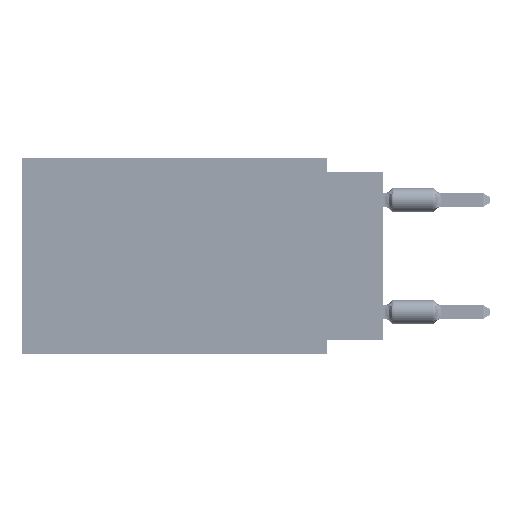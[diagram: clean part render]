
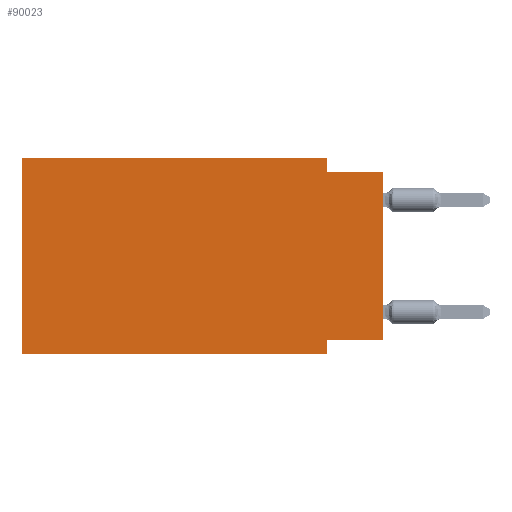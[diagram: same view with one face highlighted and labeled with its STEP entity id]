
A CAD part, left-side view. The second image highlights one B-rep face of the part: STEP entity #90023.
In plain terms, the highlighted planar face has unit normal (-1, 0, 0).
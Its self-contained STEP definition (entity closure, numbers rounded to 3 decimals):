
#874 = DIRECTION ( 'NONE',  ( 0., -1., 0. ) ) ;
#1228 = DIRECTION ( 'NONE',  ( 0., 0., 1. ) ) ;
#2649 = ORIENTED_EDGE ( 'NONE', *, *, #95040, .F. ) ;
#3822 = EDGE_CURVE ( 'NONE', #44511, #113213, #54202, .T. ) ;
#7982 = DIRECTION ( 'NONE',  ( 0., 0., -1. ) ) ;
#8481 = DIRECTION ( 'NONE',  ( 0., 0., -1. ) ) ;
#10222 = CARTESIAN_POINT ( 'NONE',  ( 0., 16.383, 0. ) ) ;
#14307 = LINE ( 'NONE', #70844, #91828 ) ;
#15457 = EDGE_CURVE ( 'NONE', #113213, #62733, #33739, .T. ) ;
#15697 = CARTESIAN_POINT ( 'NONE',  ( 0., 0., -0.635 ) ) ;
#17548 = VERTEX_POINT ( 'NONE', #62936 ) ;
#18003 = VERTEX_POINT ( 'NONE', #44712 ) ;
#18806 = PLANE ( 'NONE',  #70451 ) ;
#21100 = DIRECTION ( 'NONE',  ( 0., -1., 0. ) ) ;
#22506 = ORIENTED_EDGE ( 'NONE', *, *, #78497, .T. ) ;
#24770 = CARTESIAN_POINT ( 'NONE',  ( 0., 2.54, -8.89 ) ) ;
#27828 = FACE_OUTER_BOUND ( 'NONE', #87710, .T. ) ;
#31511 = ORIENTED_EDGE ( 'NONE', *, *, #15457, .F. ) ;
#33739 = LINE ( 'NONE', #15697, #103133 ) ;
#33762 = VERTEX_POINT ( 'NONE', #91388 ) ;
#34558 = VECTOR ( 'NONE', #21100, 1000. ) ;
#36956 = CARTESIAN_POINT ( 'NONE',  ( 0., 16.383, -8.89 ) ) ;
#39013 = VECTOR ( 'NONE', #68711, 1000. ) ;
#40032 = CARTESIAN_POINT ( 'NONE',  ( 0., 2.54, -0.635 ) ) ;
#44511 = VERTEX_POINT ( 'NONE', #113572 ) ;
#44712 = CARTESIAN_POINT ( 'NONE',  ( 0., 2.54, -8.255 ) ) ;
#47925 = ORIENTED_EDGE ( 'NONE', *, *, #105461, .F. ) ;
#52383 = DIRECTION ( 'NONE',  ( 0., -1., 0. ) ) ;
#54202 = LINE ( 'NONE', #90938, #81335 ) ;
#56422 = VERTEX_POINT ( 'NONE', #104288 ) ;
#56747 = LINE ( 'NONE', #103671, #94701 ) ;
#62733 = VERTEX_POINT ( 'NONE', #88961 ) ;
#62936 = CARTESIAN_POINT ( 'NONE',  ( 0., 16.383, 0. ) ) ;
#67404 = VECTOR ( 'NONE', #874, 1000. ) ;
#68711 = DIRECTION ( 'NONE',  ( 0., 0., -1. ) ) ;
#70451 = AXIS2_PLACEMENT_3D ( 'NONE', #91040, #72961, #7982 ) ;
#70844 = CARTESIAN_POINT ( 'NONE',  ( 0., 0., 0. ) ) ;
#72961 = DIRECTION ( 'NONE',  ( 1., 0., 0. ) ) ;
#74157 = ORIENTED_EDGE ( 'NONE', *, *, #76621, .T. ) ;
#76621 = EDGE_CURVE ( 'NONE', #56422, #33762, #82107, .T. ) ;
#78497 = EDGE_CURVE ( 'NONE', #116005, #62733, #14307, .T. ) ;
#78645 = VECTOR ( 'NONE', #1228, 1000. ) ;
#81335 = VECTOR ( 'NONE', #8481, 1000. ) ;
#82107 = LINE ( 'NONE', #36956, #67404 ) ;
#87710 = EDGE_LOOP ( 'NONE', ( #22506, #31511, #113472, #87916, #2649, #74157, #101027, #47925 ) ) ;
#87916 = ORIENTED_EDGE ( 'NONE', *, *, #116851, .F. ) ;
#88961 = CARTESIAN_POINT ( 'NONE',  ( 0., 0., -0.635 ) ) ;
#89168 = LINE ( 'NONE', #24770, #39013 ) ;
#90023 = ADVANCED_FACE ( 'NONE', ( #27828 ), #18806, .F. ) ;
#90938 = CARTESIAN_POINT ( 'NONE',  ( 0., 2.54, 0. ) ) ;
#91040 = CARTESIAN_POINT ( 'NONE',  ( 0., 16.383, 0. ) ) ;
#91388 = CARTESIAN_POINT ( 'NONE',  ( 0., 2.54, -8.89 ) ) ;
#91828 = VECTOR ( 'NONE', #107574, 1000. ) ;
#92688 = LINE ( 'NONE', #10222, #78645 ) ;
#92747 = LINE ( 'NONE', #93946, #34558 ) ;
#93946 = CARTESIAN_POINT ( 'NONE',  ( 0., 16.383, 0. ) ) ;
#94701 = VECTOR ( 'NONE', #113297, 1000. ) ;
#95040 = EDGE_CURVE ( 'NONE', #56422, #17548, #92688, .T. ) ;
#101027 = ORIENTED_EDGE ( 'NONE', *, *, #105643, .F. ) ;
#103133 = VECTOR ( 'NONE', #52383, 1000. ) ;
#103671 = CARTESIAN_POINT ( 'NONE',  ( 0., 0., -8.255 ) ) ;
#104288 = CARTESIAN_POINT ( 'NONE',  ( 0., 16.383, -8.89 ) ) ;
#105461 = EDGE_CURVE ( 'NONE', #116005, #18003, #56747, .T. ) ;
#105643 = EDGE_CURVE ( 'NONE', #18003, #33762, #89168, .T. ) ;
#107574 = DIRECTION ( 'NONE',  ( 0., 0., 1. ) ) ;
#108191 = CARTESIAN_POINT ( 'NONE',  ( 0., 0., -8.255 ) ) ;
#113213 = VERTEX_POINT ( 'NONE', #40032 ) ;
#113297 = DIRECTION ( 'NONE',  ( 0., 1., 0. ) ) ;
#113472 = ORIENTED_EDGE ( 'NONE', *, *, #3822, .F. ) ;
#113572 = CARTESIAN_POINT ( 'NONE',  ( 0., 2.54, 0. ) ) ;
#116005 = VERTEX_POINT ( 'NONE', #108191 ) ;
#116851 = EDGE_CURVE ( 'NONE', #17548, #44511, #92747, .T. ) ;
